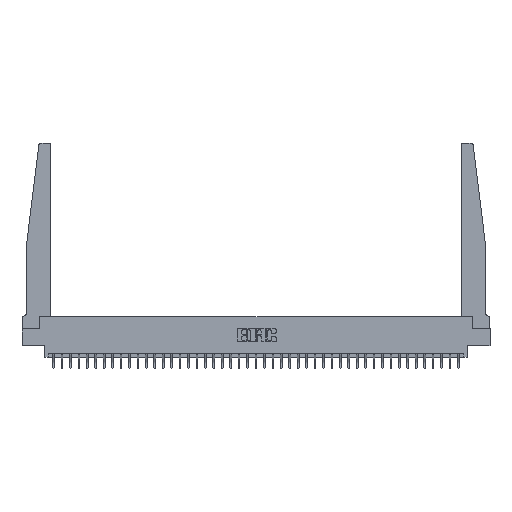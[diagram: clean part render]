
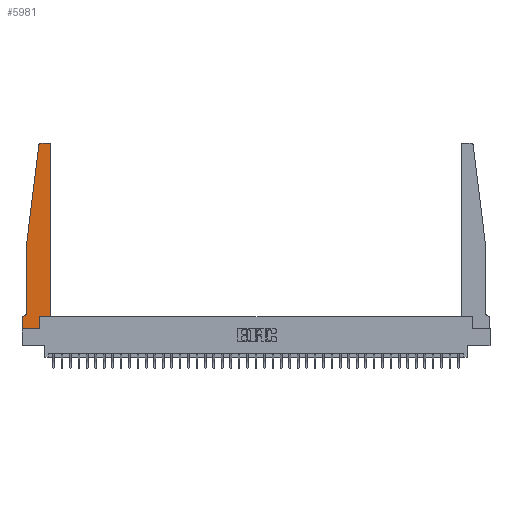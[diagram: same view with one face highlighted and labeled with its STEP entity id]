
A CAD part, top view. The second image highlights one B-rep face of the part: STEP entity #5981.
In plain terms, the highlighted planar face has unit normal (0, 0, 1).
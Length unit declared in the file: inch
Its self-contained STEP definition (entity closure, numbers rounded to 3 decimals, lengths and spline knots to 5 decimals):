
#234 = VERTEX_POINT ( 'NONE', #29300 ) ;
#358 = CARTESIAN_POINT ( 'NONE',  ( 0.015, 0.1875, 0.37 ) ) ;
#648 = CARTESIAN_POINT ( 'NONE',  ( 0.065, 1.25, 0.37 ) ) ;
#1896 = CARTESIAN_POINT ( 'NONE',  ( 0.065, 1.25, 0.37 ) ) ;
#2622 = CARTESIAN_POINT ( 'NONE',  ( 0.2605, 0.18, 0.37 ) ) ;
#2733 = CIRCLE ( 'NONE', #23058, 0.03 ) ;
#2866 = VERTEX_POINT ( 'NONE', #14997 ) ;
#3630 = LINE ( 'NONE', #648, #31607 ) ;
#5133 = DIRECTION ( 'NONE',  ( 1., 0., 0. ) ) ;
#5395 = CIRCLE ( 'NONE', #27361, 0.03 ) ;
#5441 = DIRECTION ( 'NONE',  ( 0., 1., 0. ) ) ;
#5981 = ADVANCED_FACE ( 'NONE', ( #28201 ), #19114, .T. ) ;
#6536 = CIRCLE ( 'NONE', #19211, 0.05 ) ;
#6782 = EDGE_CURVE ( 'NONE', #234, #21906, #5395, .T. ) ;
#6967 = ORIENTED_EDGE ( 'NONE', *, *, #35387, .T. ) ;
#6981 = VECTOR ( 'NONE', #5441, 39.37008 ) ;
#7266 = VERTEX_POINT ( 'NONE', #26875 ) ;
#7702 = CARTESIAN_POINT ( 'NONE',  ( 0.27653, 2.72, 0.37 ) ) ;
#7928 = ORIENTED_EDGE ( 'NONE', *, *, #18752, .T. ) ;
#8064 = EDGE_LOOP ( 'NONE', ( #6967, #28713, #32275, #32684, #7928, #12199, #24180, #9670, #28017, #14039, #12191, #22466 ) ) ;
#8518 = VECTOR ( 'NONE', #32309, 39.37008 ) ;
#9208 = DIRECTION ( 'NONE',  ( 0., 0., 1. ) ) ;
#9587 = VECTOR ( 'NONE', #13533, 39.37008 ) ;
#9670 = ORIENTED_EDGE ( 'NONE', *, *, #31642, .T. ) ;
#9952 = CARTESIAN_POINT ( 'NONE',  ( 0., 0., 0.37 ) ) ;
#10492 = DIRECTION ( 'NONE',  ( 1., 0., 0. ) ) ;
#10697 = VECTOR ( 'NONE', #34711, 39.37008 ) ;
#11771 = DIRECTION ( 'NONE',  ( 0., 1., 0. ) ) ;
#11979 = EDGE_CURVE ( 'NONE', #12712, #2866, #13927, .T. ) ;
#12191 = ORIENTED_EDGE ( 'NONE', *, *, #31816, .T. ) ;
#12199 = ORIENTED_EDGE ( 'NONE', *, *, #11979, .T. ) ;
#12712 = VERTEX_POINT ( 'NONE', #358 ) ;
#13468 = CARTESIAN_POINT ( 'NONE',  ( 0., 0.1875, 0.37 ) ) ;
#13533 = DIRECTION ( 'NONE',  ( 1., 0., 0. ) ) ;
#13592 = EDGE_CURVE ( 'NONE', #2866, #7266, #29952, .T. ) ;
#13927 = LINE ( 'NONE', #34352, #28778 ) ;
#14039 = ORIENTED_EDGE ( 'NONE', *, *, #24860, .T. ) ;
#14163 = CARTESIAN_POINT ( 'NONE',  ( 0.425, 0.18, 0.37 ) ) ;
#14552 = CARTESIAN_POINT ( 'NONE',  ( 0.015, 0.2375, 0.37 ) ) ;
#14848 = DIRECTION ( 'NONE',  ( -1., 0., 0. ) ) ;
#14997 = CARTESIAN_POINT ( 'NONE',  ( 0., 0.1875, 0.37 ) ) ;
#15314 = LINE ( 'NONE', #2622, #6981 ) ;
#16117 = CARTESIAN_POINT ( 'NONE',  ( 0.395, 2.75, 0.37 ) ) ;
#16221 = VERTEX_POINT ( 'NONE', #33281 ) ;
#16371 = CARTESIAN_POINT ( 'NONE',  ( 0., 0., 0.37 ) ) ;
#17092 = VERTEX_POINT ( 'NONE', #28964 ) ;
#17352 = DIRECTION ( 'NONE',  ( 0., -1., 0. ) ) ;
#17380 = DIRECTION ( 'NONE',  ( -1., 0., 0. ) ) ;
#17965 = VERTEX_POINT ( 'NONE', #27215 ) ;
#18373 = VECTOR ( 'NONE', #11771, 39.37008 ) ;
#18752 = EDGE_CURVE ( 'NONE', #17092, #12712, #6536, .T. ) ;
#18846 = EDGE_CURVE ( 'NONE', #35614, #24368, #2733, .T. ) ;
#19114 = PLANE ( 'NONE',  #26881 ) ;
#19211 = AXIS2_PLACEMENT_3D ( 'NONE', #14552, #34072, #17380 ) ;
#19655 = DIRECTION ( 'NONE',  ( -1., 0., 0. ) ) ;
#20419 = VERTEX_POINT ( 'NONE', #30057 ) ;
#20843 = CARTESIAN_POINT ( 'NONE',  ( 0.425, 0.18, 0.37 ) ) ;
#21728 = CARTESIAN_POINT ( 'NONE',  ( 0.24675, 2.72367, 0.37 ) ) ;
#21906 = VERTEX_POINT ( 'NONE', #21728 ) ;
#21928 = DIRECTION ( 'NONE',  ( 0., 0., 1. ) ) ;
#22033 = LINE ( 'NONE', #30594, #35944 ) ;
#22466 = ORIENTED_EDGE ( 'NONE', *, *, #18846, .T. ) ;
#23058 = AXIS2_PLACEMENT_3D ( 'NONE', #26025, #9208, #28806 ) ;
#24180 = ORIENTED_EDGE ( 'NONE', *, *, #13592, .T. ) ;
#24368 = VERTEX_POINT ( 'NONE', #16117 ) ;
#24860 = EDGE_CURVE ( 'NONE', #17965, #25959, #26497, .T. ) ;
#25535 = LINE ( 'NONE', #1896, #32029 ) ;
#25812 = LINE ( 'NONE', #31318, #18373 ) ;
#25959 = VERTEX_POINT ( 'NONE', #14163 ) ;
#26025 = CARTESIAN_POINT ( 'NONE',  ( 0.395, 2.72, 0.37 ) ) ;
#26077 = EDGE_CURVE ( 'NONE', #20419, #17092, #3630, .T. ) ;
#26497 = LINE ( 'NONE', #20843, #10697 ) ;
#26875 = CARTESIAN_POINT ( 'NONE',  ( 0., 0., 0.37 ) ) ;
#26881 = AXIS2_PLACEMENT_3D ( 'NONE', #13468, #21928, #5133 ) ;
#27215 = CARTESIAN_POINT ( 'NONE',  ( 0.2605, 0.18, 0.37 ) ) ;
#27281 = DIRECTION ( 'NONE',  ( 0., 0., 1. ) ) ;
#27361 = AXIS2_PLACEMENT_3D ( 'NONE', #7702, #27281, #10492 ) ;
#28017 = ORIENTED_EDGE ( 'NONE', *, *, #31700, .T. ) ;
#28201 = FACE_OUTER_BOUND ( 'NONE', #8064, .T. ) ;
#28713 = ORIENTED_EDGE ( 'NONE', *, *, #6782, .T. ) ;
#28778 = VECTOR ( 'NONE', #14848, 39.37008 ) ;
#28806 = DIRECTION ( 'NONE',  ( 1., 0., 0. ) ) ;
#28964 = CARTESIAN_POINT ( 'NONE',  ( 0.065, 0.2375, 0.37 ) ) ;
#29300 = CARTESIAN_POINT ( 'NONE',  ( 0.27653, 2.75, 0.37 ) ) ;
#29952 = LINE ( 'NONE', #9952, #8518 ) ;
#30057 = CARTESIAN_POINT ( 'NONE',  ( 0.065, 1.25, 0.37 ) ) ;
#30594 = CARTESIAN_POINT ( 'NONE',  ( 0.25, 2.75, 0.37 ) ) ;
#31318 = CARTESIAN_POINT ( 'NONE',  ( 0.425, 0.18, 0.37 ) ) ;
#31607 = VECTOR ( 'NONE', #17352, 39.37008 ) ;
#31642 = EDGE_CURVE ( 'NONE', #7266, #16221, #32762, .T. ) ;
#31676 = CARTESIAN_POINT ( 'NONE',  ( 0.425, 2.72, 0.37 ) ) ;
#31700 = EDGE_CURVE ( 'NONE', #16221, #17965, #15314, .T. ) ;
#31816 = EDGE_CURVE ( 'NONE', #25959, #35614, #25812, .T. ) ;
#32029 = VECTOR ( 'NONE', #32698, 39.37008 ) ;
#32275 = ORIENTED_EDGE ( 'NONE', *, *, #35968, .T. ) ;
#32309 = DIRECTION ( 'NONE',  ( 0., -1., 0. ) ) ;
#32684 = ORIENTED_EDGE ( 'NONE', *, *, #26077, .T. ) ;
#32698 = DIRECTION ( 'NONE',  ( -0.122, -0.992, 0. ) ) ;
#32762 = LINE ( 'NONE', #16371, #9587 ) ;
#33281 = CARTESIAN_POINT ( 'NONE',  ( 0.2605, 0., 0.37 ) ) ;
#34072 = DIRECTION ( 'NONE',  ( 0., 0., -1. ) ) ;
#34352 = CARTESIAN_POINT ( 'NONE',  ( 0.065, 0.1875, 0.37 ) ) ;
#34711 = DIRECTION ( 'NONE',  ( 1., 0., 0. ) ) ;
#35387 = EDGE_CURVE ( 'NONE', #24368, #234, #22033, .T. ) ;
#35614 = VERTEX_POINT ( 'NONE', #31676 ) ;
#35944 = VECTOR ( 'NONE', #19655, 39.37008 ) ;
#35968 = EDGE_CURVE ( 'NONE', #21906, #20419, #25535, .T. ) ;
